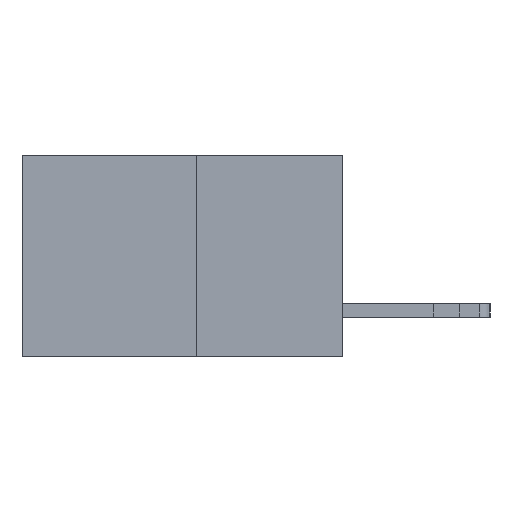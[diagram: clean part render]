
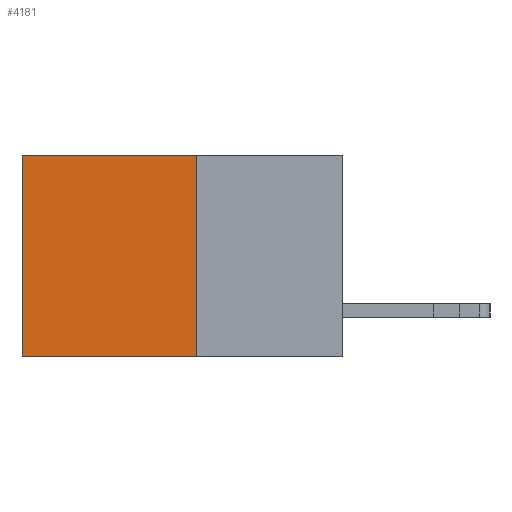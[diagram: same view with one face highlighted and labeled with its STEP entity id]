
A CAD part, left-side view. The second image highlights one B-rep face of the part: STEP entity #4181.
In plain terms, the highlighted planar face has unit normal (-1, 0, 0).
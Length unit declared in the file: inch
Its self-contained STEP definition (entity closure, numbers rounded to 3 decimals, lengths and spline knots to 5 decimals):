
#1469 = DIRECTION ( 'NONE',  ( 0., 0., -1. ) ) ;
#4181 = ADVANCED_FACE ( 'NONE', ( #8537 ), #11571, .F. ) ;
#4317 = VERTEX_POINT ( 'NONE', #5713 ) ;
#4382 = VERTEX_POINT ( 'NONE', #12942 ) ;
#4543 = EDGE_LOOP ( 'NONE', ( #7262, #5761, #18618, #6294 ) ) ;
#4726 = VECTOR ( 'NONE', #7642, 39.37008 ) ;
#5713 = CARTESIAN_POINT ( 'NONE',  ( 0.277, 0.27, -0.37 ) ) ;
#5761 = ORIENTED_EDGE ( 'NONE', *, *, #9638, .F. ) ;
#6293 = DIRECTION ( 'NONE',  ( 0., 0., -1. ) ) ;
#6294 = ORIENTED_EDGE ( 'NONE', *, *, #11585, .T. ) ;
#7262 = ORIENTED_EDGE ( 'NONE', *, *, #11337, .T. ) ;
#7269 = VECTOR ( 'NONE', #1469, 39.37008 ) ;
#7642 = DIRECTION ( 'NONE',  ( 0., 1., 0. ) ) ;
#8164 = DIRECTION ( 'NONE',  ( 0., 0., -1. ) ) ;
#8537 = FACE_OUTER_BOUND ( 'NONE', #4543, .T. ) ;
#8551 = LINE ( 'NONE', #11941, #4726 ) ;
#9495 = AXIS2_PLACEMENT_3D ( 'NONE', #11073, #14956, #8164 ) ;
#9638 = EDGE_CURVE ( 'NONE', #4317, #18235, #8551, .T. ) ;
#10838 = VECTOR ( 'NONE', #6293, 39.37008 ) ;
#11073 = CARTESIAN_POINT ( 'NONE',  ( 0.277, 0.27, -0.37 ) ) ;
#11337 = EDGE_CURVE ( 'NONE', #4382, #18235, #17995, .T. ) ;
#11571 = PLANE ( 'NONE',  #9495 ) ;
#11585 = EDGE_CURVE ( 'NONE', #17817, #4382, #13986, .T. ) ;
#11696 = CARTESIAN_POINT ( 'NONE',  ( 0.277, 0.27, -0.37 ) ) ;
#11941 = CARTESIAN_POINT ( 'NONE',  ( 0.277, 0.27, -0.37 ) ) ;
#12846 = CARTESIAN_POINT ( 'NONE',  ( 0.277, 0.27, 0. ) ) ;
#12942 = CARTESIAN_POINT ( 'NONE',  ( 0.277, 0.59, 0. ) ) ;
#13986 = LINE ( 'NONE', #14002, #17766 ) ;
#14002 = CARTESIAN_POINT ( 'NONE',  ( 0.277, 0.27, 0. ) ) ;
#14956 = DIRECTION ( 'NONE',  ( 1., 0., 0. ) ) ;
#14976 = CARTESIAN_POINT ( 'NONE',  ( 0.277, 0.59, -0.37 ) ) ;
#14992 = LINE ( 'NONE', #11696, #7269 ) ;
#15215 = CARTESIAN_POINT ( 'NONE',  ( 0.277, 0.59, -0.37 ) ) ;
#15461 = DIRECTION ( 'NONE',  ( 0., 1., 0. ) ) ;
#17766 = VECTOR ( 'NONE', #15461, 39.37008 ) ;
#17817 = VERTEX_POINT ( 'NONE', #12846 ) ;
#17995 = LINE ( 'NONE', #14976, #10838 ) ;
#18235 = VERTEX_POINT ( 'NONE', #15215 ) ;
#18618 = ORIENTED_EDGE ( 'NONE', *, *, #18632, .F. ) ;
#18632 = EDGE_CURVE ( 'NONE', #17817, #4317, #14992, .T. ) ;
